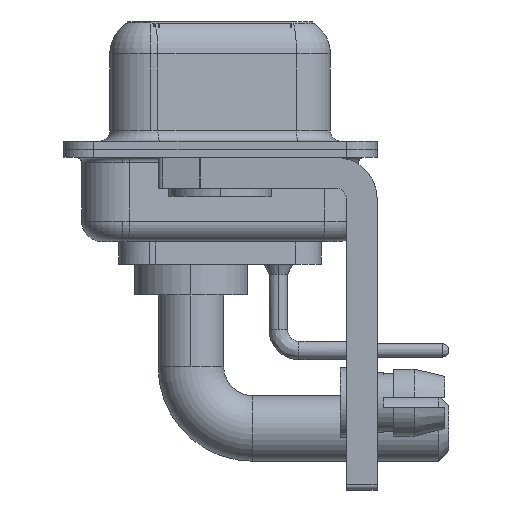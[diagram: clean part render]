
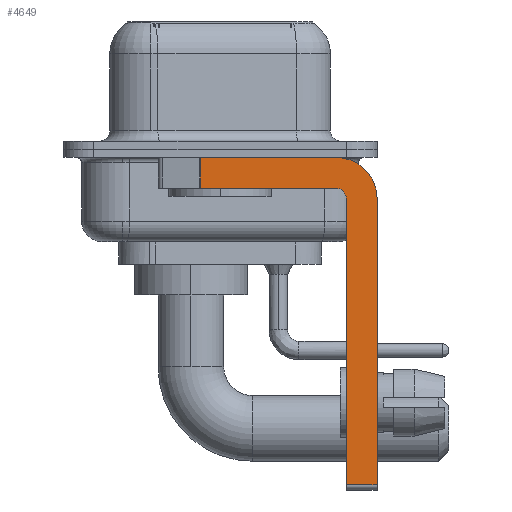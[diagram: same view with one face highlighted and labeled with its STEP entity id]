
A CAD part, left-side view. The second image highlights one B-rep face of the part: STEP entity #4649.
In plain terms, the highlighted planar face has unit normal (-1, 0, 0).
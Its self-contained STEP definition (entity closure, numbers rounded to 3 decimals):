
#68 = VERTEX_POINT ( 'NONE', #439 ) ;
#212 = EDGE_CURVE ( 'NONE', #17502, #15387, #19293, .T. ) ;
#432 = EDGE_CURVE ( 'NONE', #16473, #17227, #19270, .T. ) ;
#439 = CARTESIAN_POINT ( 'NONE',  ( -2.9, -7.65, -2.4 ) ) ;
#1183 = VERTEX_POINT ( 'NONE', #3538 ) ;
#1245 = DIRECTION ( 'NONE',  ( 0., -1., 0. ) ) ;
#1281 = CARTESIAN_POINT ( 'NONE',  ( -2.9, -5.65, -1.9 ) ) ;
#1463 = LINE ( 'NONE', #15676, #3902 ) ;
#1555 = DIRECTION ( 'NONE',  ( 0., 0., 1. ) ) ;
#1741 = EDGE_CURVE ( 'NONE', #16473, #6882, #10213, .T. ) ;
#2134 = AXIS2_PLACEMENT_3D ( 'NONE', #5369, #8840, #1555 ) ;
#2572 = EDGE_CURVE ( 'NONE', #17502, #1183, #3219, .T. ) ;
#2576 = VECTOR ( 'NONE', #23223, 1000. ) ;
#3157 = VECTOR ( 'NONE', #4637, 1000. ) ;
#3219 = LINE ( 'NONE', #23016, #3157 ) ;
#3451 = EDGE_CURVE ( 'NONE', #68, #6882, #1463, .T. ) ;
#3538 = CARTESIAN_POINT ( 'NONE',  ( -2.9, 0.978, -1.9 ) ) ;
#3562 = CARTESIAN_POINT ( 'NONE',  ( -2.9, -5.65, -2.4 ) ) ;
#3902 = VECTOR ( 'NONE', #10189, 1000. ) ;
#4371 = AXIS2_PLACEMENT_3D ( 'NONE', #3562, #14547, #21817 ) ;
#4637 = DIRECTION ( 'NONE',  ( 0., 0., -1. ) ) ;
#4642 = VECTOR ( 'NONE', #1245, 1000. ) ;
#4649 = ADVANCED_FACE ( 'NONE', ( #5354 ), #12659, .F. ) ;
#4898 = CARTESIAN_POINT ( 'NONE',  ( -2.9, -5.65, -2.4 ) ) ;
#4928 = VECTOR ( 'NONE', #6162, 1000. ) ;
#5185 = CARTESIAN_POINT ( 'NONE',  ( -2.9, -5.65, -16.35 ) ) ;
#5354 = FACE_OUTER_BOUND ( 'NONE', #16741, .T. ) ;
#5369 = CARTESIAN_POINT ( 'NONE',  ( -2.9, -5.65, -2.4 ) ) ;
#5716 = VECTOR ( 'NONE', #12123, 1000. ) ;
#6162 = DIRECTION ( 'NONE',  ( 0., -1., 0. ) ) ;
#6426 = EDGE_CURVE ( 'NONE', #6512, #1183, #23463, .T. ) ;
#6512 = VERTEX_POINT ( 'NONE', #14644 ) ;
#6882 = VERTEX_POINT ( 'NONE', #23558 ) ;
#8244 = DIRECTION ( 'NONE',  ( 0., 0., -1. ) ) ;
#8606 = ORIENTED_EDGE ( 'NONE', *, *, #3451, .F. ) ;
#8715 = ORIENTED_EDGE ( 'NONE', *, *, #432, .F. ) ;
#8840 = DIRECTION ( 'NONE',  ( -1., 0., 0. ) ) ;
#8954 = ORIENTED_EDGE ( 'NONE', *, *, #15397, .F. ) ;
#9608 = AXIS2_PLACEMENT_3D ( 'NONE', #4898, #10279, #8244 ) ;
#10189 = DIRECTION ( 'NONE',  ( 0., 0., -1. ) ) ;
#10213 = LINE ( 'NONE', #5185, #4642 ) ;
#10279 = DIRECTION ( 'NONE',  ( 1., 0., 0. ) ) ;
#10342 = CARTESIAN_POINT ( 'NONE',  ( -2.9, 3., -0.4 ) ) ;
#10633 = ORIENTED_EDGE ( 'NONE', *, *, #2572, .T. ) ;
#10639 = CARTESIAN_POINT ( 'NONE',  ( -2.9, -5.65, -0.4 ) ) ;
#12123 = DIRECTION ( 'NONE',  ( 0., 0., 1. ) ) ;
#12659 = PLANE ( 'NONE',  #4371 ) ;
#12834 = CARTESIAN_POINT ( 'NONE',  ( -2.9, -6.15, -16.35 ) ) ;
#13667 = CARTESIAN_POINT ( 'NONE',  ( -2.9, 0.978, -0.4 ) ) ;
#13900 = CARTESIAN_POINT ( 'NONE',  ( -2.9, -6.15, -16.6 ) ) ;
#14547 = DIRECTION ( 'NONE',  ( 1., 0., 0. ) ) ;
#14644 = CARTESIAN_POINT ( 'NONE',  ( -2.9, -5.65, -1.9 ) ) ;
#14999 = CIRCLE ( 'NONE', #9608, 2. ) ;
#15387 = VERTEX_POINT ( 'NONE', #10639 ) ;
#15397 = EDGE_CURVE ( 'NONE', #17227, #6512, #22686, .T. ) ;
#15676 = CARTESIAN_POINT ( 'NONE',  ( -2.9, -7.65, -2.4 ) ) ;
#15926 = ORIENTED_EDGE ( 'NONE', *, *, #6426, .F. ) ;
#16473 = VERTEX_POINT ( 'NONE', #12834 ) ;
#16741 = EDGE_LOOP ( 'NONE', ( #17580, #10633, #15926, #8954, #8715, #21412, #8606, #23450 ) ) ;
#17227 = VERTEX_POINT ( 'NONE', #17863 ) ;
#17502 = VERTEX_POINT ( 'NONE', #13667 ) ;
#17580 = ORIENTED_EDGE ( 'NONE', *, *, #212, .F. ) ;
#17863 = CARTESIAN_POINT ( 'NONE',  ( -2.9, -6.15, -2.4 ) ) ;
#19270 = LINE ( 'NONE', #13900, #5716 ) ;
#19293 = LINE ( 'NONE', #10342, #4928 ) ;
#21153 = EDGE_CURVE ( 'NONE', #15387, #68, #14999, .T. ) ;
#21412 = ORIENTED_EDGE ( 'NONE', *, *, #1741, .T. ) ;
#21817 = DIRECTION ( 'NONE',  ( 0., 0., -1. ) ) ;
#22686 = CIRCLE ( 'NONE', #2134, 0.5 ) ;
#23016 = CARTESIAN_POINT ( 'NONE',  ( -2.9, 0.978, -1.9 ) ) ;
#23223 = DIRECTION ( 'NONE',  ( 0., 1., 0. ) ) ;
#23450 = ORIENTED_EDGE ( 'NONE', *, *, #21153, .F. ) ;
#23463 = LINE ( 'NONE', #1281, #2576 ) ;
#23558 = CARTESIAN_POINT ( 'NONE',  ( -2.9, -7.65, -16.35 ) ) ;
